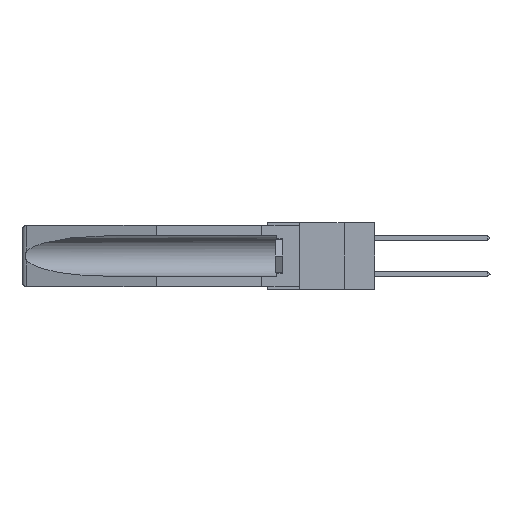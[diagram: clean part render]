
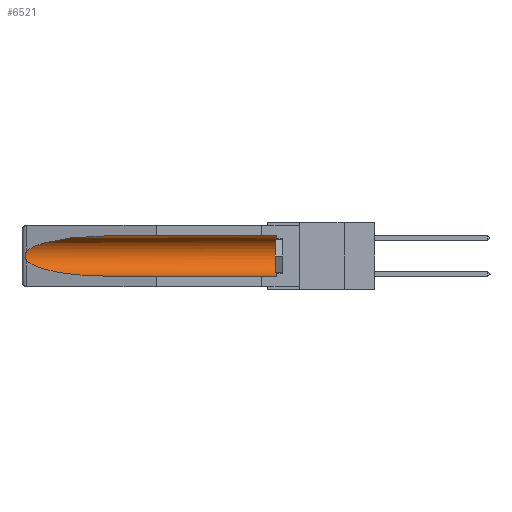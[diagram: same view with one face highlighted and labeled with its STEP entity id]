
A CAD part, left-side view. The second image highlights one B-rep face of the part: STEP entity #6521.
In plain terms, the highlighted cylindrical face has radius 2.857 mm (diameter 5.715 mm), a partial arc.
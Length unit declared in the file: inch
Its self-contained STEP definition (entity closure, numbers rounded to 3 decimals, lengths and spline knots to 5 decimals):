
#147 = VERTEX_POINT ( 'NONE', #4162 ) ;
#493 = CARTESIAN_POINT ( 'NONE',  ( 0.26537, 1.52718, -0.19328 ) ) ;
#765 = CARTESIAN_POINT ( 'NONE',  ( 0.26537, 1.52718, -0.14972 ) ) ;
#1062 = FACE_OUTER_BOUND ( 'NONE', #16213, .T. ) ;
#1861 = ORIENTED_EDGE ( 'NONE', *, *, #3549, .T. ) ;
#1899 = VERTEX_POINT ( 'NONE', #493 ) ;
#2093 = EDGE_CURVE ( 'NONE', #19600, #1899, #17532, .T. ) ;
#2591 = CIRCLE ( 'NONE', #6339, 0.1125 ) ;
#2691 =( BOUNDED_CURVE ( )  B_SPLINE_CURVE ( 3, ( #19820, #19753, #13568, #5563 ),
 .UNSPECIFIED., .F., .F. ) 
 B_SPLINE_CURVE_WITH_KNOTS ( ( 4, 4 ),
 ( 0.1948, 1.5708 ),
 .UNSPECIFIED. ) 
 CURVE ( )  GEOMETRIC_REPRESENTATION_ITEM ( )  RATIONAL_B_SPLINE_CURVE ( ( 1., 0.848, 0.848, 1. ) ) 
 REPRESENTATION_ITEM ( '' )  );
#2695 = CARTESIAN_POINT ( 'NONE',  ( 0.26537, 1.52718, -0.14972 ) ) ;
#2833 = CARTESIAN_POINT ( 'NONE',  ( 0.2673, 1.53269, -0.17917 ) ) ;
#2894 = VERTEX_POINT ( 'NONE', #6856 ) ;
#3088 = EDGE_CURVE ( 'NONE', #2894, #147, #17221, .T. ) ;
#3549 = EDGE_CURVE ( 'NONE', #11746, #11752, #8886, .T. ) ;
#3706 = VECTOR ( 'NONE', #5392, 39.37008 ) ;
#4162 = CARTESIAN_POINT ( 'NONE',  ( 0.155, 1.07973, -0.284 ) ) ;
#4332 = CARTESIAN_POINT ( 'NONE',  ( 0.26597, 1.52961, -0.15275 ) ) ;
#4678 = CARTESIAN_POINT ( 'NONE',  ( 0.155, 1.07973, -0.059 ) ) ;
#4872 = ORIENTED_EDGE ( 'NONE', *, *, #2093, .T. ) ;
#5350 = CARTESIAN_POINT ( 'NONE',  ( 0.155, -0.30754, -0.1715 ) ) ;
#5392 = DIRECTION ( 'NONE',  ( 0., 1., 0. ) ) ;
#5563 = CARTESIAN_POINT ( 'NONE',  ( 0.155, 1.07973, -0.284 ) ) ;
#5793 = DIRECTION ( 'NONE',  ( 0., 1., 0. ) ) ;
#6065 = CARTESIAN_POINT ( 'NONE',  ( 0.21114, 1.30732, -0.059 ) ) ;
#6339 = AXIS2_PLACEMENT_3D ( 'NONE', #10696, #9255, #15361 ) ;
#6521 = ADVANCED_FACE ( 'NONE', ( #1062 ), #17267, .F. ) ;
#6635 = EDGE_CURVE ( 'NONE', #1899, #147, #2691, .T. ) ;
#6745 = ORIENTED_EDGE ( 'NONE', *, *, #17825, .T. ) ;
#6856 = CARTESIAN_POINT ( 'NONE',  ( 0.155, 0.126, -0.284 ) ) ;
#7377 = CARTESIAN_POINT ( 'NONE',  ( 0.155, -0.30754, -0.059 ) ) ;
#7431 = CARTESIAN_POINT ( 'NONE',  ( 0.26655, 1.53094, -0.18657 ) ) ;
#7502 = CARTESIAN_POINT ( 'NONE',  ( 0.2673, 1.5327, -0.16383 ) ) ;
#8533 = DIRECTION ( 'NONE',  ( 0., 0., 1. ) ) ;
#8886 = LINE ( 'NONE', #7377, #11061 ) ;
#8957 = CARTESIAN_POINT ( 'NONE',  ( 0.2675, 1.53308, -0.17534 ) ) ;
#9154 = CARTESIAN_POINT ( 'NONE',  ( 0.25451, 1.48313, -0.09465 ) ) ;
#9255 = DIRECTION ( 'NONE',  ( 0., -1., 0. ) ) ;
#10525 = CARTESIAN_POINT ( 'NONE',  ( 0.26537, 1.52718, -0.19328 ) ) ;
#10696 = CARTESIAN_POINT ( 'NONE',  ( 0.155, 0.126, -0.1715 ) ) ;
#11061 = VECTOR ( 'NONE', #5793, 39.37008 ) ;
#11746 = VERTEX_POINT ( 'NONE', #16388 ) ;
#11752 = VERTEX_POINT ( 'NONE', #13146 ) ;
#12226 = CARTESIAN_POINT ( 'NONE',  ( 0.26654, 1.53092, -0.15636 ) ) ;
#13146 = CARTESIAN_POINT ( 'NONE',  ( 0.155, 1.07973, -0.059 ) ) ;
#13308 = AXIS2_PLACEMENT_3D ( 'NONE', #5350, #14750, #8533 ) ;
#13433 = ORIENTED_EDGE ( 'NONE', *, *, #3088, .F. ) ;
#13568 = CARTESIAN_POINT ( 'NONE',  ( 0.21114, 1.30732, -0.284 ) ) ;
#13662 = CARTESIAN_POINT ( 'NONE',  ( 0.2675, 1.53308, -0.16763 ) ) ;
#14750 = DIRECTION ( 'NONE',  ( 0., 1., 0. ) ) ;
#14846 = EDGE_CURVE ( 'NONE', #2894, #11746, #2591, .T. ) ;
#15361 = DIRECTION ( 'NONE',  ( 0., 0., 1. ) ) ;
#16213 = EDGE_LOOP ( 'NONE', ( #6745, #4872, #19143, #13433, #16747, #1861 ) ) ;
#16388 = CARTESIAN_POINT ( 'NONE',  ( 0.155, 0.126, -0.059 ) ) ;
#16747 = ORIENTED_EDGE ( 'NONE', *, *, #14846, .T. ) ;
#17156 = CARTESIAN_POINT ( 'NONE',  ( 0.26537, 1.52718, -0.14972 ) ) ;
#17221 = LINE ( 'NONE', #19601, #3706 ) ;
#17267 = CYLINDRICAL_SURFACE ( 'NONE', #13308, 0.1125 ) ;
#17532 = B_SPLINE_CURVE_WITH_KNOTS ( 'NONE', 3,
 ( #2695, #4332, #12226, #7502, #13662, #8957, #2833, #7431, #19907, #10525 ),
 .UNSPECIFIED., .F., .F.,
 ( 4, 2, 2, 2, 4 ),
 ( 0., 0.00029, 0.00058, 0.00087, 0.00117 ),
 .UNSPECIFIED. ) ;
#17825 = EDGE_CURVE ( 'NONE', #11752, #19600, #18799, .T. ) ;
#18799 =( BOUNDED_CURVE ( )  B_SPLINE_CURVE ( 3, ( #4678, #6065, #9154, #17156 ),
 .UNSPECIFIED., .F., .F. ) 
 B_SPLINE_CURVE_WITH_KNOTS ( ( 4, 4 ),
 ( 4.71239, 6.08839 ),
 .UNSPECIFIED. ) 
 CURVE ( )  GEOMETRIC_REPRESENTATION_ITEM ( )  RATIONAL_B_SPLINE_CURVE ( ( 1., 0.848, 0.848, 1. ) ) 
 REPRESENTATION_ITEM ( '' )  );
#19143 = ORIENTED_EDGE ( 'NONE', *, *, #6635, .T. ) ;
#19600 = VERTEX_POINT ( 'NONE', #765 ) ;
#19601 = CARTESIAN_POINT ( 'NONE',  ( 0.155, -0.30754, -0.284 ) ) ;
#19753 = CARTESIAN_POINT ( 'NONE',  ( 0.25451, 1.48313, -0.24835 ) ) ;
#19820 = CARTESIAN_POINT ( 'NONE',  ( 0.26537, 1.52718, -0.19328 ) ) ;
#19907 = CARTESIAN_POINT ( 'NONE',  ( 0.26597, 1.5296, -0.19026 ) ) ;
